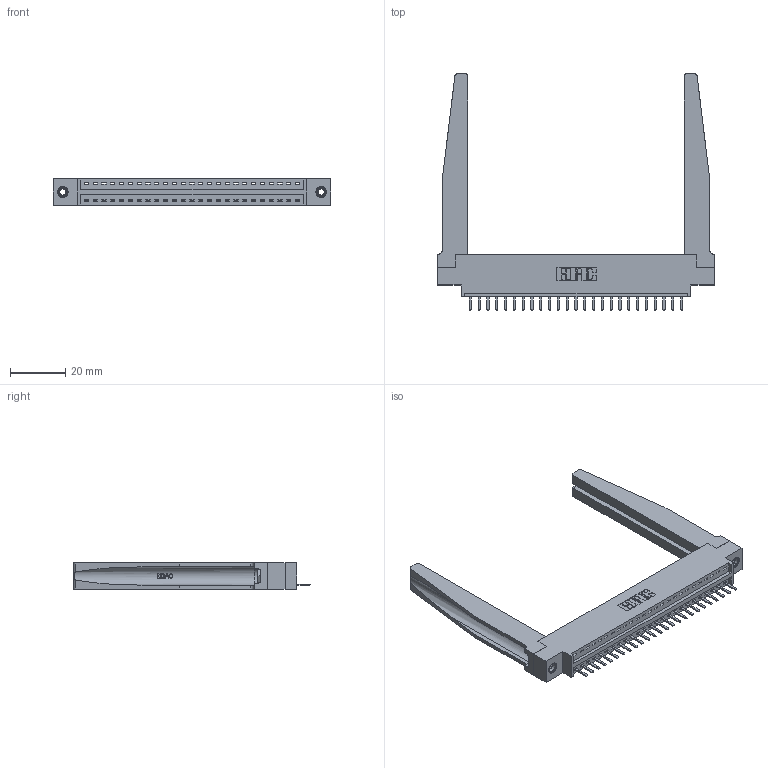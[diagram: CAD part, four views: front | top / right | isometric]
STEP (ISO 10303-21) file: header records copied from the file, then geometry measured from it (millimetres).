
FILE_DESCRIPTION (( 'STEP AP203' ), '1' );
FILE_NAME ('396-025-520-678.STEP', '2019-10-27T06:17:35', ( '' ), ( '' ), 'SwSTEP 2.0', 'SolidWorks 2016', '' );
FILE_SCHEMA (( 'CONFIG_CONTROL_DESIGN' ));
Length unit declared in the file: inch
Products named in the file (5): 346-220-078_345-220-078; 345-292-001_345-293-120; 396-025-520-678; 345-250-001_345-250-001-102; 346 Part_0.170 Offset - 0.156 Dia-TH
Assembly tree (30 placements, depth 2):
  396-025-520-678
    346 Part_0.170 Offset - 0.156 Dia-TH
    345-292-001_345-293-120  x25
    346-220-078_345-220-078  x2
    345-250-001_345-250-001-102  x2
Bounding box: 99.95 x 85.29 x 9.4 mm (x, y, z)
Volume: 16132.5 mm3; surface area: 17805.3 mm2
Topology: 30 solids, 30 shells, 1910 faces, 5549 edges, 3622 vertices
Faces by surface type: plane 1272, cylinder 586, bspline 36, cone 12, torus 4
Entity records: 22798 total; most frequent: CARTESIAN_POINT 4838, ORIENTED_EDGE 3674, DIRECTION 3261, EDGE_CURVE 1837, LINE 1507, VECTOR 1507, VERTEX_POINT 1216, AXIS2_PLACEMENT_3D 877
